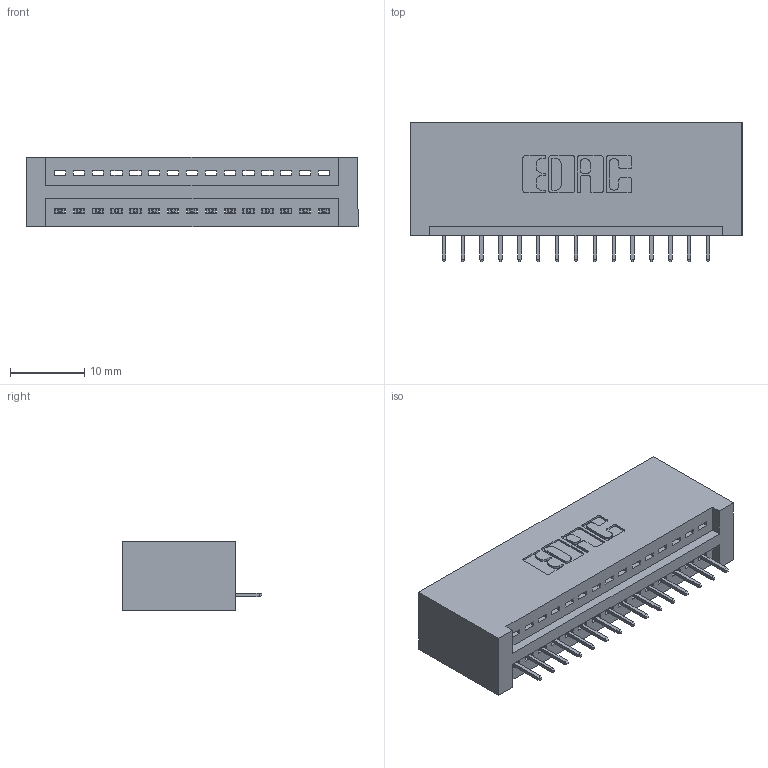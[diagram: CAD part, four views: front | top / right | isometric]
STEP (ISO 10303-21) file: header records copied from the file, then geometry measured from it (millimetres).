
FILE_DESCRIPTION (( 'STEP AP203' ), '1' );
FILE_NAME ('845-015-525-101.STEP', '2020-09-22T18:02:41', ( '' ), ( '' ), 'SwSTEP 2.0', 'SolidWorks 2020', '' );
FILE_SCHEMA (( 'CONFIG_CONTROL_DESIGN' ));
Length unit declared in the file: inch
Products named in the file (3): 345-292-001_345-293-125; 845-015-525-101; 845 Part_No Mounting Lugs
Assembly tree (16 placements, depth 2):
  845-015-525-101
    845 Part_No Mounting Lugs
    345-292-001_345-293-125  x15
Bounding box: 44.7 x 18.72 x 9.4 mm (x, y, z)
Volume: 4548 mm3; surface area: 5662.8 mm2
Topology: 16 solids, 16 shells, 1048 faces, 3017 edges, 1950 vertices
Faces by surface type: plane 766, cylinder 282
Entity records: 14721 total; most frequent: CARTESIAN_POINT 2557, ORIENTED_EDGE 2506, DIRECTION 2267, EDGE_CURVE 1253, LINE 1073, VECTOR 1073, VERTEX_POINT 830, AXIS2_PLACEMENT_3D 597
